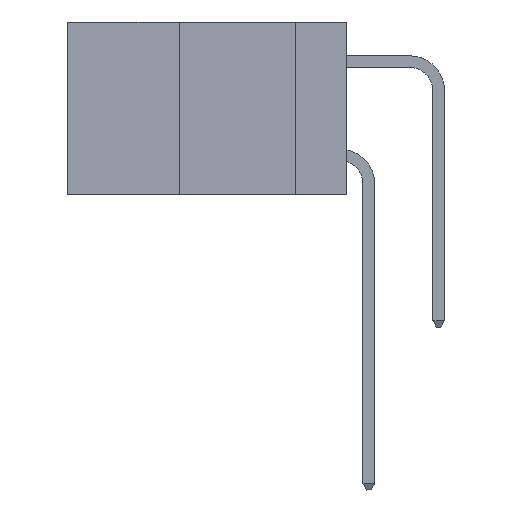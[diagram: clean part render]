
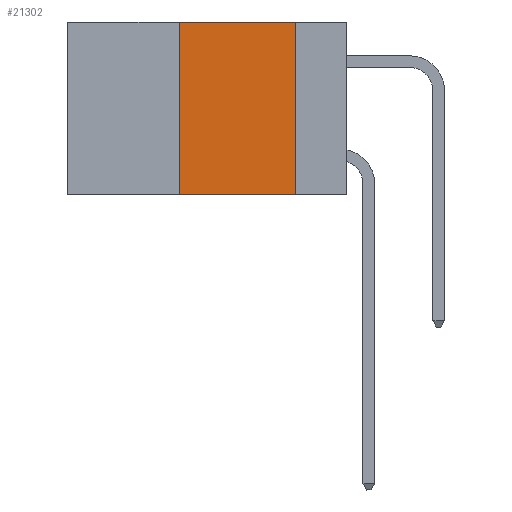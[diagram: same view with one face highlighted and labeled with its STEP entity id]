
A CAD part, left-side view. The second image highlights one B-rep face of the part: STEP entity #21302.
In plain terms, the highlighted planar face has unit normal (-1, 0, 0).
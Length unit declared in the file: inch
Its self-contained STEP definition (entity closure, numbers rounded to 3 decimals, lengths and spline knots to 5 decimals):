
#185 = CARTESIAN_POINT ( 'NONE',  ( 0., 0.11, 0. ) ) ;
#1670 = CARTESIAN_POINT ( 'NONE',  ( 0., 0.6, 0. ) ) ;
#1989 = EDGE_CURVE ( 'NONE', #5415, #5806, #9634, .T. ) ;
#2634 = ORIENTED_EDGE ( 'NONE', *, *, #16919, .F. ) ;
#2754 = PLANE ( 'NONE',  #4244 ) ;
#2812 = LINE ( 'NONE', #2999, #9411 ) ;
#2999 = CARTESIAN_POINT ( 'NONE',  ( 0., 0.36, 0. ) ) ;
#3801 = CARTESIAN_POINT ( 'NONE',  ( 0., 0.36, -0.37 ) ) ;
#4244 = AXIS2_PLACEMENT_3D ( 'NONE', #19112, #9686, #5878 ) ;
#5276 = VECTOR ( 'NONE', #8446, 39.37008 ) ;
#5415 = VERTEX_POINT ( 'NONE', #3801 ) ;
#5806 = VERTEX_POINT ( 'NONE', #18889 ) ;
#5820 = EDGE_CURVE ( 'NONE', #5415, #25555, #2812, .T. ) ;
#5878 = DIRECTION ( 'NONE',  ( 0., 0., -1. ) ) ;
#5998 = EDGE_LOOP ( 'NONE', ( #9124, #2634, #13359, #19499 ) ) ;
#7484 = DIRECTION ( 'NONE',  ( 0., 0., -1. ) ) ;
#8446 = DIRECTION ( 'NONE',  ( 0., -1., 0. ) ) ;
#8989 = VECTOR ( 'NONE', #13399, 39.37008 ) ;
#9124 = ORIENTED_EDGE ( 'NONE', *, *, #14905, .F. ) ;
#9411 = VECTOR ( 'NONE', #20714, 39.37008 ) ;
#9634 = LINE ( 'NONE', #17449, #8989 ) ;
#9686 = DIRECTION ( 'NONE',  ( 1., 0., 0. ) ) ;
#10096 = VECTOR ( 'NONE', #7484, 39.37008 ) ;
#10593 = LINE ( 'NONE', #1670, #5276 ) ;
#13359 = ORIENTED_EDGE ( 'NONE', *, *, #5820, .F. ) ;
#13399 = DIRECTION ( 'NONE',  ( 0., -1., 0. ) ) ;
#14601 = FACE_OUTER_BOUND ( 'NONE', #5998, .T. ) ;
#14905 = EDGE_CURVE ( 'NONE', #20216, #5806, #19349, .T. ) ;
#15375 = CARTESIAN_POINT ( 'NONE',  ( 0., 0.11, 0. ) ) ;
#16919 = EDGE_CURVE ( 'NONE', #25555, #20216, #10593, .T. ) ;
#17449 = CARTESIAN_POINT ( 'NONE',  ( 0., 0.6, -0.37 ) ) ;
#18889 = CARTESIAN_POINT ( 'NONE',  ( 0., 0.11, -0.37 ) ) ;
#19112 = CARTESIAN_POINT ( 'NONE',  ( 0., 0.6, 0. ) ) ;
#19349 = LINE ( 'NONE', #15375, #10096 ) ;
#19499 = ORIENTED_EDGE ( 'NONE', *, *, #1989, .T. ) ;
#20216 = VERTEX_POINT ( 'NONE', #185 ) ;
#20714 = DIRECTION ( 'NONE',  ( 0., 0., 1. ) ) ;
#21302 = ADVANCED_FACE ( 'NONE', ( #14601 ), #2754, .F. ) ;
#22366 = CARTESIAN_POINT ( 'NONE',  ( 0., 0.36, 0. ) ) ;
#25555 = VERTEX_POINT ( 'NONE', #22366 ) ;
